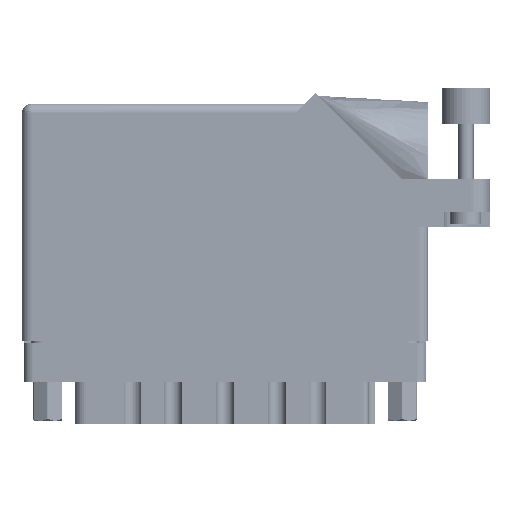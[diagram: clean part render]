
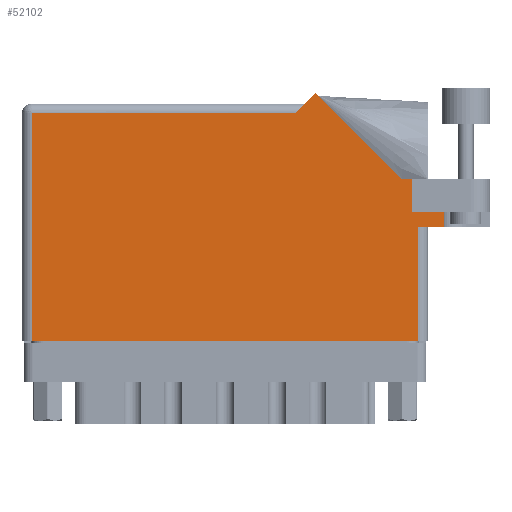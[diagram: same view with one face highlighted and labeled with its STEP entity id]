
A CAD part, front view. The second image highlights one B-rep face of the part: STEP entity #52102.
In plain terms, the highlighted face is planar.
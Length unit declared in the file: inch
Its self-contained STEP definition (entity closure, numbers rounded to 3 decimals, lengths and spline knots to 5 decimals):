
#317 = EDGE_CURVE ( 'NONE', #43580, #40800, #20864, .T. ) ;
#383 = CARTESIAN_POINT ( 'NONE',  ( 2.44642, 1.044, 0. ) ) ;
#562 = VECTOR ( 'NONE', #21488, 39.37008 ) ;
#2173 = CARTESIAN_POINT ( 'NONE',  ( 2.512, 0.831, 0. ) ) ;
#2228 = CARTESIAN_POINT ( 'NONE',  ( 0.062, 0., 0. ) ) ;
#2382 = DIRECTION ( 'NONE',  ( 0., -1., 0. ) ) ;
#2584 = VERTEX_POINT ( 'NONE', #2173 ) ;
#2616 = CARTESIAN_POINT ( 'NONE',  ( 0., 1.468, 0. ) ) ;
#5171 = LINE ( 'NONE', #21241, #38434 ) ;
#5215 = CARTESIAN_POINT ( 'NONE',  ( 2.7135, 1.16177, 0. ) ) ;
#6216 = ORIENTED_EDGE ( 'NONE', *, *, #32619, .T. ) ;
#6295 = EDGE_LOOP ( 'NONE', ( #46461, #50933, #53770, #38182, #13158, #12529, #11518, #40223, #12177, #45119, #6216 ) ) ;
#6898 = CARTESIAN_POINT ( 'NONE',  ( 1.819, 1.53, 0. ) ) ;
#8153 = EDGE_CURVE ( 'NONE', #54498, #58698, #5171, .T. ) ;
#9080 = VECTOR ( 'NONE', #53664, 39.37008 ) ;
#9875 = VECTOR ( 'NONE', #2382, 39.37008 ) ;
#10745 = VERTEX_POINT ( 'NONE', #19580 ) ;
#11493 = VECTOR ( 'NONE', #12129, 39.37008 ) ;
#11518 = ORIENTED_EDGE ( 'NONE', *, *, #33226, .T. ) ;
#12054 = PLANE ( 'NONE',  #30314 ) ;
#12129 = DIRECTION ( 'NONE',  ( -1., 0., 0. ) ) ;
#12177 = ORIENTED_EDGE ( 'NONE', *, *, #45312, .T. ) ;
#12529 = ORIENTED_EDGE ( 'NONE', *, *, #42021, .T. ) ;
#13158 = ORIENTED_EDGE ( 'NONE', *, *, #37524, .F. ) ;
#13449 = CARTESIAN_POINT ( 'NONE',  ( 2.7135, 0.737, 0. ) ) ;
#13955 = VERTEX_POINT ( 'NONE', #56372 ) ;
#14289 = DIRECTION ( 'NONE',  ( 0., 1., 0. ) ) ;
#15184 = VECTOR ( 'NONE', #55832, 39.37008 ) ;
#16271 = VERTEX_POINT ( 'NONE', #18146 ) ;
#16468 = DIRECTION ( 'NONE',  ( 0., 0., -1. ) ) ;
#17662 = VERTEX_POINT ( 'NONE', #22387 ) ;
#18146 = CARTESIAN_POINT ( 'NONE',  ( 1.88971, 1.60071, 0. ) ) ;
#18880 = EDGE_CURVE ( 'NONE', #58698, #51145, #49786, .T. ) ;
#19580 = CARTESIAN_POINT ( 'NONE',  ( 0.062, 1.468, 0. ) ) ;
#20864 = LINE ( 'NONE', #5215, #61692 ) ;
#20935 = DIRECTION ( 'NONE',  ( -1., 0., 0. ) ) ;
#21031 = LINE ( 'NONE', #55345, #562 ) ;
#21241 = CARTESIAN_POINT ( 'NONE',  ( 0., 0., 0. ) ) ;
#21488 = DIRECTION ( 'NONE',  ( -1., 0., 0. ) ) ;
#21764 = LINE ( 'NONE', #6898, #23982 ) ;
#21970 = CARTESIAN_POINT ( 'NONE',  ( 2.44642, 1.044, 0. ) ) ;
#22387 = CARTESIAN_POINT ( 'NONE',  ( 2.512, 1.044, 0. ) ) ;
#22747 = LINE ( 'NONE', #31351, #9875 ) ;
#23982 = VECTOR ( 'NONE', #46216, 39.37008 ) ;
#25056 = DIRECTION ( 'NONE',  ( 1., 0., 0. ) ) ;
#26482 = DIRECTION ( 'NONE',  ( 1., 0., 0. ) ) ;
#28918 = CARTESIAN_POINT ( 'NONE',  ( 2.7135, 0.831, 0. ) ) ;
#30314 = AXIS2_PLACEMENT_3D ( 'NONE', #50517, #16468, #20935 ) ;
#31351 = CARTESIAN_POINT ( 'NONE',  ( 0.062, 0., 0. ) ) ;
#31694 = VECTOR ( 'NONE', #39898, 39.37008 ) ;
#32109 = VERTEX_POINT ( 'NONE', #383 ) ;
#32619 = EDGE_CURVE ( 'NONE', #10745, #54498, #22747, .T. ) ;
#33041 = EDGE_CURVE ( 'NONE', #51145, #40800, #60518, .T. ) ;
#33226 = EDGE_CURVE ( 'NONE', #17662, #32109, #21031, .T. ) ;
#33576 = CARTESIAN_POINT ( 'NONE',  ( 2.612, 0.737, 0. ) ) ;
#34338 = DIRECTION ( 'NONE',  ( 0., -1., 0. ) ) ;
#35871 = CARTESIAN_POINT ( 'NONE',  ( 2.55, 0.737, 0. ) ) ;
#37524 = EDGE_CURVE ( 'NONE', #2584, #43580, #55795, .T. ) ;
#38182 = ORIENTED_EDGE ( 'NONE', *, *, #317, .F. ) ;
#38434 = VECTOR ( 'NONE', #26482, 39.37008 ) ;
#39898 = DIRECTION ( 'NONE',  ( 0., 1., 0. ) ) ;
#40223 = ORIENTED_EDGE ( 'NONE', *, *, #57508, .T. ) ;
#40800 = VERTEX_POINT ( 'NONE', #13449 ) ;
#40920 = FACE_OUTER_BOUND ( 'NONE', #6295, .T. ) ;
#41507 = CARTESIAN_POINT ( 'NONE',  ( 2.55, 0., 0. ) ) ;
#42021 = EDGE_CURVE ( 'NONE', #2584, #17662, #46092, .T. ) ;
#43580 = VERTEX_POINT ( 'NONE', #28918 ) ;
#45119 = ORIENTED_EDGE ( 'NONE', *, *, #58535, .T. ) ;
#45312 = EDGE_CURVE ( 'NONE', #16271, #13955, #21764, .T. ) ;
#46092 = LINE ( 'NONE', #54296, #31694 ) ;
#46216 = DIRECTION ( 'NONE',  ( -0.707, -0.707, 0. ) ) ;
#46461 = ORIENTED_EDGE ( 'NONE', *, *, #8153, .T. ) ;
#48580 = CARTESIAN_POINT ( 'NONE',  ( 2.512, 0.831, 0. ) ) ;
#48976 = VECTOR ( 'NONE', #25056, 39.37008 ) ;
#49786 = LINE ( 'NONE', #58279, #54287 ) ;
#50517 = CARTESIAN_POINT ( 'NONE',  ( 0., 1.53, 0. ) ) ;
#50933 = ORIENTED_EDGE ( 'NONE', *, *, #18880, .T. ) ;
#51145 = VERTEX_POINT ( 'NONE', #35871 ) ;
#52102 = ADVANCED_FACE ( 'NONE', ( #40920 ), #12054, .F. ) ;
#53664 = DIRECTION ( 'NONE',  ( 1., 0., 0. ) ) ;
#53770 = ORIENTED_EDGE ( 'NONE', *, *, #33041, .T. ) ;
#53839 = LINE ( 'NONE', #2616, #11493 ) ;
#54287 = VECTOR ( 'NONE', #14289, 39.37008 ) ;
#54296 = CARTESIAN_POINT ( 'NONE',  ( 2.512, 0.831, 0. ) ) ;
#54498 = VERTEX_POINT ( 'NONE', #2228 ) ;
#55345 = CARTESIAN_POINT ( 'NONE',  ( 3.012, 1.044, 0. ) ) ;
#55795 = LINE ( 'NONE', #48580, #48976 ) ;
#55832 = DIRECTION ( 'NONE',  ( -0.707, 0.707, 0. ) ) ;
#56372 = CARTESIAN_POINT ( 'NONE',  ( 1.757, 1.468, 0. ) ) ;
#57508 = EDGE_CURVE ( 'NONE', #32109, #16271, #59093, .T. ) ;
#58279 = CARTESIAN_POINT ( 'NONE',  ( 2.55, 0.737, 0. ) ) ;
#58535 = EDGE_CURVE ( 'NONE', #13955, #10745, #53839, .T. ) ;
#58698 = VERTEX_POINT ( 'NONE', #41507 ) ;
#59093 = LINE ( 'NONE', #21970, #15184 ) ;
#60518 = LINE ( 'NONE', #33576, #9080 ) ;
#61692 = VECTOR ( 'NONE', #34338, 39.37008 ) ;
